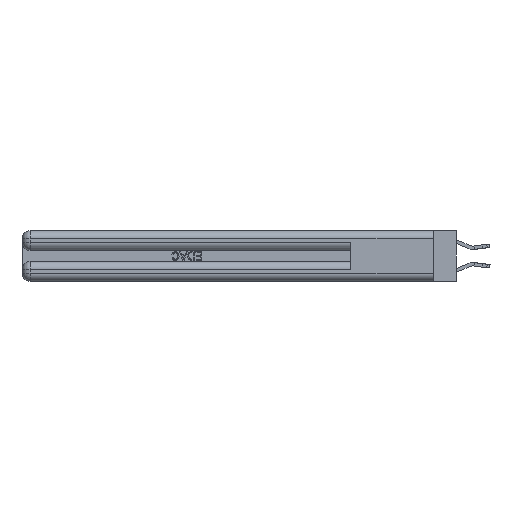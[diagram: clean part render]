
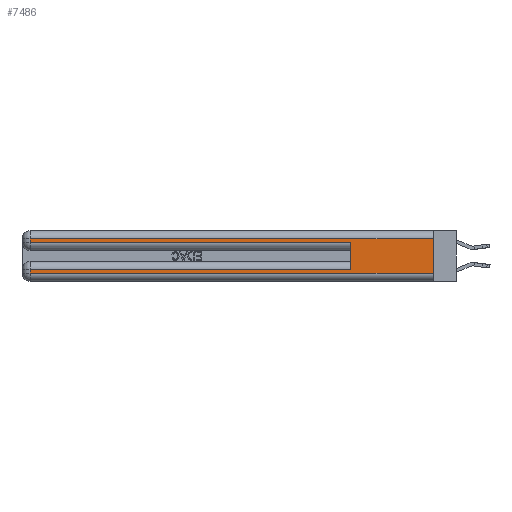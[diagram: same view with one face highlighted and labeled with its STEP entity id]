
A CAD part, left-side view. The second image highlights one B-rep face of the part: STEP entity #7486.
In plain terms, the highlighted planar face has unit normal (-1, 0, 0).
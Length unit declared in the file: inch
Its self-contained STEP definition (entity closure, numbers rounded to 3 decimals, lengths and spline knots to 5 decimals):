
#233 = ORIENTED_EDGE ( 'NONE', *, *, #10464, .T. ) ;
#753 = CARTESIAN_POINT ( 'NONE',  ( 0., 0., 0.06 ) ) ;
#1104 = CARTESIAN_POINT ( 'NONE',  ( 0., 2.94, 0.37 ) ) ;
#1135 = CARTESIAN_POINT ( 'NONE',  ( 0., 2.94, 0.285 ) ) ;
#1182 = FACE_OUTER_BOUND ( 'NONE', #22200, .T. ) ;
#1474 = LINE ( 'NONE', #3702, #20169 ) ;
#1550 = DIRECTION ( 'NONE',  ( 0., 0., -1. ) ) ;
#1788 = VERTEX_POINT ( 'NONE', #29708 ) ;
#2520 = LINE ( 'NONE', #1104, #8268 ) ;
#3702 = CARTESIAN_POINT ( 'NONE',  ( 0., 0.6, 0.145 ) ) ;
#4512 = DIRECTION ( 'NONE',  ( 0., 1., 0. ) ) ;
#4631 = CARTESIAN_POINT ( 'NONE',  ( 0., 2.94, 0.31 ) ) ;
#5113 = VECTOR ( 'NONE', #23489, 39.37008 ) ;
#5220 = ORIENTED_EDGE ( 'NONE', *, *, #21876, .F. ) ;
#5719 = CARTESIAN_POINT ( 'NONE',  ( 0., 0.6, 0.285 ) ) ;
#5954 = DIRECTION ( 'NONE',  ( 0., -1., 0. ) ) ;
#6852 = EDGE_CURVE ( 'NONE', #19126, #15931, #9235, .T. ) ;
#7228 = VERTEX_POINT ( 'NONE', #10320 ) ;
#7486 = ADVANCED_FACE ( 'NONE', ( #1182 ), #30677, .F. ) ;
#7512 = LINE ( 'NONE', #23920, #14012 ) ;
#7977 = LINE ( 'NONE', #10746, #20182 ) ;
#8268 = VECTOR ( 'NONE', #13371, 39.37008 ) ;
#9235 = LINE ( 'NONE', #30399, #27892 ) ;
#10320 = CARTESIAN_POINT ( 'NONE',  ( 0., 2.94, 0.085 ) ) ;
#10464 = EDGE_CURVE ( 'NONE', #1788, #7228, #7512, .T. ) ;
#10746 = CARTESIAN_POINT ( 'NONE',  ( 0., 0., 0.285 ) ) ;
#12137 = VECTOR ( 'NONE', #25646, 39.37008 ) ;
#12366 = EDGE_CURVE ( 'NONE', #19126, #30801, #28343, .T. ) ;
#13371 = DIRECTION ( 'NONE',  ( 0., 0., -1. ) ) ;
#13422 = DIRECTION ( 'NONE',  ( 0., 0., -1. ) ) ;
#13711 = CARTESIAN_POINT ( 'NONE',  ( 0., 0., 0.37 ) ) ;
#14012 = VECTOR ( 'NONE', #19058, 39.37008 ) ;
#14017 = EDGE_CURVE ( 'NONE', #30801, #19713, #18114, .T. ) ;
#14754 = ORIENTED_EDGE ( 'NONE', *, *, #27725, .T. ) ;
#14776 = CARTESIAN_POINT ( 'NONE',  ( 0., 2.94, 0.06 ) ) ;
#15851 = CARTESIAN_POINT ( 'NONE',  ( 0., 0., 0.06 ) ) ;
#15859 = DIRECTION ( 'NONE',  ( 0., 0., 1. ) ) ;
#15931 = VERTEX_POINT ( 'NONE', #753 ) ;
#16150 = DIRECTION ( 'NONE',  ( 1., 0., 0. ) ) ;
#16672 = CARTESIAN_POINT ( 'NONE',  ( 0., 0., 0.31 ) ) ;
#16996 = VERTEX_POINT ( 'NONE', #14776 ) ;
#18114 = LINE ( 'NONE', #18632, #5113 ) ;
#18632 = CARTESIAN_POINT ( 'NONE',  ( 0., 2.94, 0.37 ) ) ;
#18667 = LINE ( 'NONE', #15851, #12137 ) ;
#19058 = DIRECTION ( 'NONE',  ( 0., 1., 0. ) ) ;
#19126 = VERTEX_POINT ( 'NONE', #27688 ) ;
#19704 = ORIENTED_EDGE ( 'NONE', *, *, #29309, .T. ) ;
#19713 = VERTEX_POINT ( 'NONE', #1135 ) ;
#20169 = VECTOR ( 'NONE', #15859, 39.37008 ) ;
#20182 = VECTOR ( 'NONE', #5954, 39.37008 ) ;
#20367 = VECTOR ( 'NONE', #4512, 39.37008 ) ;
#21268 = ORIENTED_EDGE ( 'NONE', *, *, #12366, .T. ) ;
#21876 = EDGE_CURVE ( 'NONE', #1788, #31107, #1474, .T. ) ;
#22200 = EDGE_LOOP ( 'NONE', ( #27316, #21268, #24692, #28106, #5220, #233, #19704, #14754 ) ) ;
#23288 = AXIS2_PLACEMENT_3D ( 'NONE', #13711, #16150, #1550 ) ;
#23489 = DIRECTION ( 'NONE',  ( 0., 0., -1. ) ) ;
#23920 = CARTESIAN_POINT ( 'NONE',  ( 0., 0., 0.085 ) ) ;
#24692 = ORIENTED_EDGE ( 'NONE', *, *, #14017, .T. ) ;
#25646 = DIRECTION ( 'NONE',  ( 0., -1., 0. ) ) ;
#27316 = ORIENTED_EDGE ( 'NONE', *, *, #6852, .F. ) ;
#27674 = EDGE_CURVE ( 'NONE', #19713, #31107, #7977, .T. ) ;
#27688 = CARTESIAN_POINT ( 'NONE',  ( 0., 0., 0.31 ) ) ;
#27725 = EDGE_CURVE ( 'NONE', #16996, #15931, #18667, .T. ) ;
#27892 = VECTOR ( 'NONE', #13422, 39.37008 ) ;
#28106 = ORIENTED_EDGE ( 'NONE', *, *, #27674, .T. ) ;
#28343 = LINE ( 'NONE', #16672, #20367 ) ;
#29309 = EDGE_CURVE ( 'NONE', #7228, #16996, #2520, .T. ) ;
#29708 = CARTESIAN_POINT ( 'NONE',  ( 0., 0.6, 0.085 ) ) ;
#30399 = CARTESIAN_POINT ( 'NONE',  ( 0., 0., 0.37 ) ) ;
#30677 = PLANE ( 'NONE',  #23288 ) ;
#30801 = VERTEX_POINT ( 'NONE', #4631 ) ;
#31107 = VERTEX_POINT ( 'NONE', #5719 ) ;
